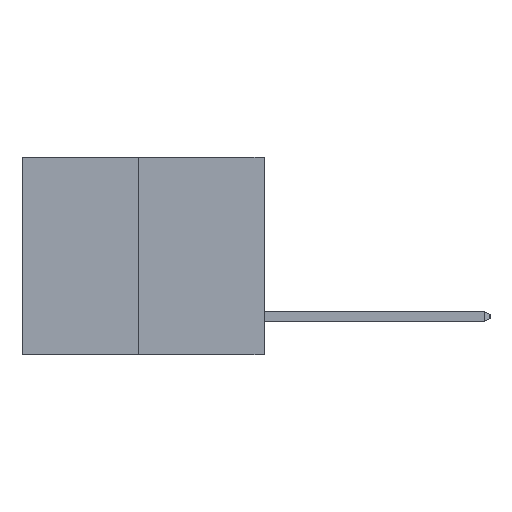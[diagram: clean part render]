
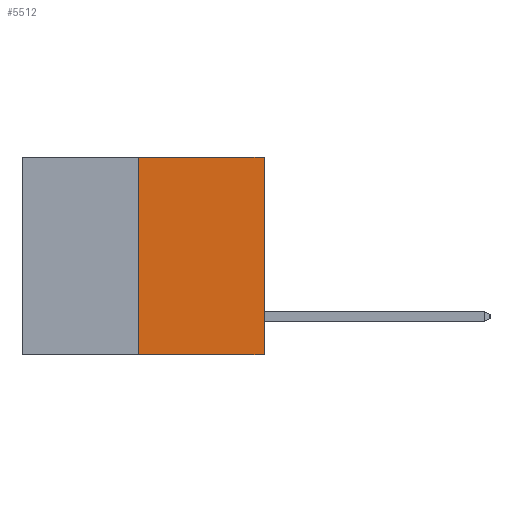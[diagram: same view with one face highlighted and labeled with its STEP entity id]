
A CAD part, left-side view. The second image highlights one B-rep face of the part: STEP entity #5512.
In plain terms, the highlighted planar face has unit normal (-1, 0, 0).
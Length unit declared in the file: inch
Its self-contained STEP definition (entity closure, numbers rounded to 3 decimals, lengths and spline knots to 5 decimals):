
#71 = VECTOR ( 'NONE', #10802, 39.37008 ) ;
#97 = VECTOR ( 'NONE', #3710, 39.37008 ) ;
#1538 = LINE ( 'NONE', #9593, #3709 ) ;
#1682 = CARTESIAN_POINT ( 'NONE',  ( 0., 0., -0.49 ) ) ;
#2174 = CARTESIAN_POINT ( 'NONE',  ( 0., 0.312, -0.49 ) ) ;
#3709 = VECTOR ( 'NONE', #5861, 39.37008 ) ;
#3710 = DIRECTION ( 'NONE',  ( 0., 0., 1. ) ) ;
#4025 = ORIENTED_EDGE ( 'NONE', *, *, #8155, .F. ) ;
#4308 = CARTESIAN_POINT ( 'NONE',  ( 0., 0., 0. ) ) ;
#4359 = ORIENTED_EDGE ( 'NONE', *, *, #6039, .T. ) ;
#4683 = CARTESIAN_POINT ( 'NONE',  ( 0., 0.312, -0.49 ) ) ;
#4741 = ORIENTED_EDGE ( 'NONE', *, *, #5582, .F. ) ;
#4867 = LINE ( 'NONE', #2174, #97 ) ;
#5512 = ADVANCED_FACE ( 'NONE', ( #9924 ), #9278, .F. ) ;
#5582 = EDGE_CURVE ( 'NONE', #5812, #11863, #4867, .T. ) ;
#5812 = VERTEX_POINT ( 'NONE', #4683 ) ;
#5861 = DIRECTION ( 'NONE',  ( 0., -1., 0. ) ) ;
#6039 = EDGE_CURVE ( 'NONE', #5812, #6693, #1538, .T. ) ;
#6058 = EDGE_LOOP ( 'NONE', ( #4741, #4359, #9567, #4025 ) ) ;
#6693 = VERTEX_POINT ( 'NONE', #1682 ) ;
#6991 = CARTESIAN_POINT ( 'NONE',  ( 0., 0.6, 0. ) ) ;
#7049 = VERTEX_POINT ( 'NONE', #9428 ) ;
#7384 = DIRECTION ( 'NONE',  ( 0., 0., -1. ) ) ;
#7504 = CARTESIAN_POINT ( 'NONE',  ( 0., 0.312, 0. ) ) ;
#8031 = LINE ( 'NONE', #6991, #71 ) ;
#8155 = EDGE_CURVE ( 'NONE', #11863, #7049, #8031, .T. ) ;
#9278 = PLANE ( 'NONE',  #11334 ) ;
#9428 = CARTESIAN_POINT ( 'NONE',  ( 0., 0., 0. ) ) ;
#9459 = EDGE_CURVE ( 'NONE', #6693, #7049, #11444, .T. ) ;
#9567 = ORIENTED_EDGE ( 'NONE', *, *, #9459, .T. ) ;
#9593 = CARTESIAN_POINT ( 'NONE',  ( 0., 0.6, -0.49 ) ) ;
#9924 = FACE_OUTER_BOUND ( 'NONE', #6058, .T. ) ;
#10480 = DIRECTION ( 'NONE',  ( 1., 0., 0. ) ) ;
#10753 = DIRECTION ( 'NONE',  ( 0., 0., 1. ) ) ;
#10802 = DIRECTION ( 'NONE',  ( 0., -1., 0. ) ) ;
#10869 = VECTOR ( 'NONE', #10753, 39.37008 ) ;
#11077 = CARTESIAN_POINT ( 'NONE',  ( 0., 0.6, 0. ) ) ;
#11334 = AXIS2_PLACEMENT_3D ( 'NONE', #11077, #10480, #7384 ) ;
#11444 = LINE ( 'NONE', #4308, #10869 ) ;
#11863 = VERTEX_POINT ( 'NONE', #7504 ) ;
